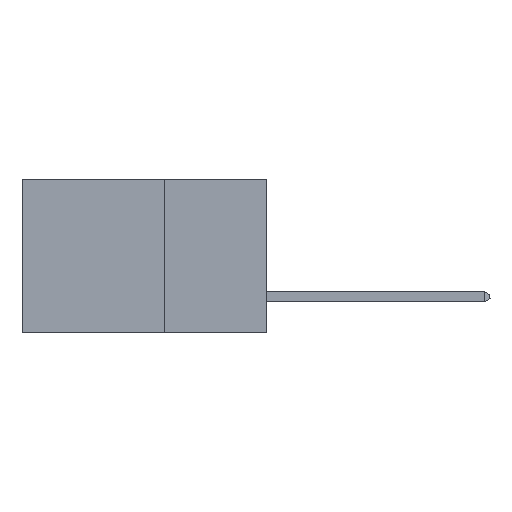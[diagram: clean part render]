
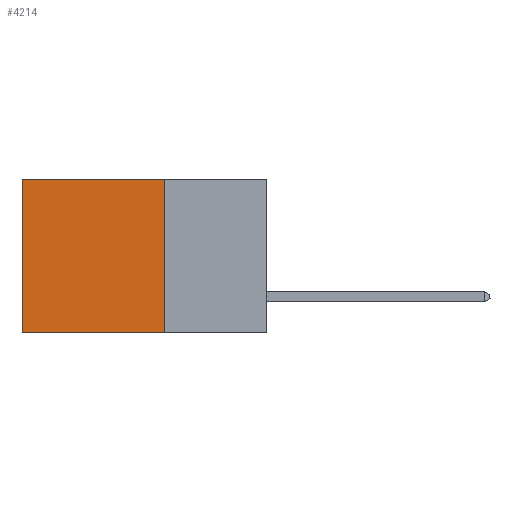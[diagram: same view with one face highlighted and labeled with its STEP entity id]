
A CAD part, left-side view. The second image highlights one B-rep face of the part: STEP entity #4214.
In plain terms, the highlighted planar face has unit normal (-1, 0, 0).
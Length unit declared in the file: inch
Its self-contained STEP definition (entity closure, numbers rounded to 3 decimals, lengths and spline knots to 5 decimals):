
#575 = DIRECTION ( 'NONE',  ( 1., 0., 0. ) ) ;
#770 = LINE ( 'NONE', #3943, #15085 ) ;
#1595 = LINE ( 'NONE', #1664, #15039 ) ;
#1664 = CARTESIAN_POINT ( 'NONE',  ( 0.2875, 0.25, 0. ) ) ;
#1772 = CARTESIAN_POINT ( 'NONE',  ( 0.2875, 0.6, 0. ) ) ;
#1811 = VECTOR ( 'NONE', #2911, 39.37008 ) ;
#2716 = ORIENTED_EDGE ( 'NONE', *, *, #11532, .T. ) ;
#2890 = EDGE_CURVE ( 'NONE', #12333, #14898, #1595, .T. ) ;
#2911 = DIRECTION ( 'NONE',  ( 0., 0., -1. ) ) ;
#3391 = VECTOR ( 'NONE', #15202, 39.37008 ) ;
#3393 = CARTESIAN_POINT ( 'NONE',  ( 0.2875, 0.25, -0.375 ) ) ;
#3943 = CARTESIAN_POINT ( 'NONE',  ( 0.2875, 0.25, -0.375 ) ) ;
#4214 = ADVANCED_FACE ( 'NONE', ( #8277 ), #17179, .F. ) ;
#4482 = CARTESIAN_POINT ( 'NONE',  ( 0.2875, 0.25, 0. ) ) ;
#4846 = DIRECTION ( 'NONE',  ( 0., 0., -1. ) ) ;
#6400 = CARTESIAN_POINT ( 'NONE',  ( 0.2875, 0.6, -0.375 ) ) ;
#6978 = ORIENTED_EDGE ( 'NONE', *, *, #8871, .F. ) ;
#7871 = DIRECTION ( 'NONE',  ( 0., 1., 0. ) ) ;
#8097 = CARTESIAN_POINT ( 'NONE',  ( 0.2875, 0.25, -0.375 ) ) ;
#8277 = FACE_OUTER_BOUND ( 'NONE', #15567, .T. ) ;
#8871 = EDGE_CURVE ( 'NONE', #12333, #13049, #17432, .T. ) ;
#9379 = CARTESIAN_POINT ( 'NONE',  ( 0.2875, 0.6, -0.375 ) ) ;
#11194 = CARTESIAN_POINT ( 'NONE',  ( 0.2875, 0.25, -0.375 ) ) ;
#11532 = EDGE_CURVE ( 'NONE', #14898, #12929, #16221, .T. ) ;
#12333 = VERTEX_POINT ( 'NONE', #4482 ) ;
#12491 = EDGE_CURVE ( 'NONE', #13049, #12929, #770, .T. ) ;
#12929 = VERTEX_POINT ( 'NONE', #6400 ) ;
#13049 = VERTEX_POINT ( 'NONE', #8097 ) ;
#13071 = AXIS2_PLACEMENT_3D ( 'NONE', #3393, #575, #4846 ) ;
#13256 = ORIENTED_EDGE ( 'NONE', *, *, #2890, .T. ) ;
#14898 = VERTEX_POINT ( 'NONE', #1772 ) ;
#15039 = VECTOR ( 'NONE', #15428, 39.37008 ) ;
#15085 = VECTOR ( 'NONE', #7871, 39.37008 ) ;
#15202 = DIRECTION ( 'NONE',  ( 0., 0., -1. ) ) ;
#15428 = DIRECTION ( 'NONE',  ( 0., 1., 0. ) ) ;
#15567 = EDGE_LOOP ( 'NONE', ( #2716, #17891, #6978, #13256 ) ) ;
#16221 = LINE ( 'NONE', #9379, #3391 ) ;
#17179 = PLANE ( 'NONE',  #13071 ) ;
#17432 = LINE ( 'NONE', #11194, #1811 ) ;
#17891 = ORIENTED_EDGE ( 'NONE', *, *, #12491, .F. ) ;
